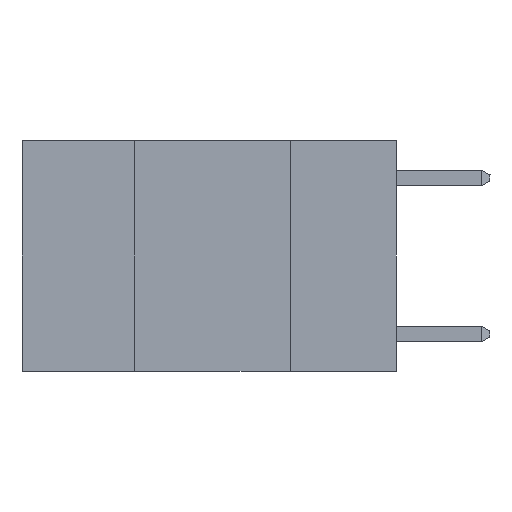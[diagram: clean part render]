
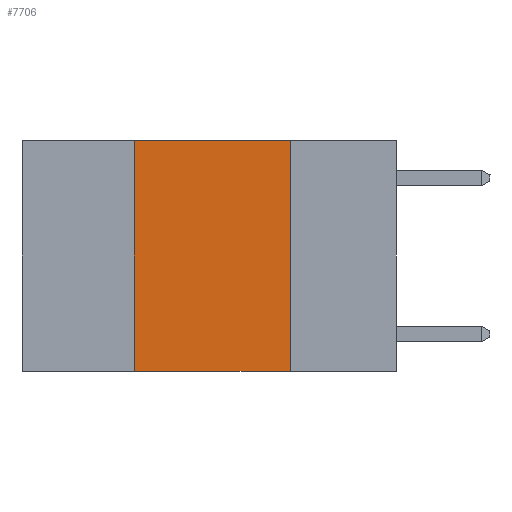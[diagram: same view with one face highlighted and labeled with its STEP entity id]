
A CAD part, left-side view. The second image highlights one B-rep face of the part: STEP entity #7706.
In plain terms, the highlighted planar face has unit normal (-1, 0, 0).
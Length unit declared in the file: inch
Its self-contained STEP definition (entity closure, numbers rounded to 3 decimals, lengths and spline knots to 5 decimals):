
#62 = ORIENTED_EDGE ( 'NONE', *, *, #2070, .F. ) ;
#86 = CARTESIAN_POINT ( 'NONE',  ( 0., 0.6, -0.37 ) ) ;
#140 = PLANE ( 'NONE',  #3904 ) ;
#459 = DIRECTION ( 'NONE',  ( 0., -1., 0. ) ) ;
#2070 = EDGE_CURVE ( 'NONE', #9289, #2929, #2936, .T. ) ;
#2397 = FACE_OUTER_BOUND ( 'NONE', #9527, .T. ) ;
#2909 = VECTOR ( 'NONE', #459, 39.37008 ) ;
#2929 = VERTEX_POINT ( 'NONE', #5144 ) ;
#2933 = CARTESIAN_POINT ( 'NONE',  ( 0., 0.6, 0. ) ) ;
#2936 = LINE ( 'NONE', #5142, #5556 ) ;
#3004 = EDGE_CURVE ( 'NONE', #8438, #9289, #6847, .T. ) ;
#3589 = EDGE_CURVE ( 'NONE', #9292, #2929, #6780, .T. ) ;
#3771 = DIRECTION ( 'NONE',  ( 0., 0., -1. ) ) ;
#3900 = DIRECTION ( 'NONE',  ( 0., -1., 0. ) ) ;
#3904 = AXIS2_PLACEMENT_3D ( 'NONE', #2933, #5977, #8201 ) ;
#3919 = ORIENTED_EDGE ( 'NONE', *, *, #3589, .T. ) ;
#4177 = ORIENTED_EDGE ( 'NONE', *, *, #8016, .F. ) ;
#4740 = CARTESIAN_POINT ( 'NONE',  ( 0., 0.6, 0. ) ) ;
#4844 = VECTOR ( 'NONE', #8734, 39.37008 ) ;
#5080 = CARTESIAN_POINT ( 'NONE',  ( 0., 0.17, 0. ) ) ;
#5142 = CARTESIAN_POINT ( 'NONE',  ( 0., 0.17, 0. ) ) ;
#5144 = CARTESIAN_POINT ( 'NONE',  ( 0., 0.17, -0.37 ) ) ;
#5285 = VECTOR ( 'NONE', #3900, 39.37008 ) ;
#5556 = VECTOR ( 'NONE', #3771, 39.37008 ) ;
#5977 = DIRECTION ( 'NONE',  ( 1., 0., 0. ) ) ;
#6107 = CARTESIAN_POINT ( 'NONE',  ( 0., 0.42, 0. ) ) ;
#6584 = CARTESIAN_POINT ( 'NONE',  ( 0., 0.42, 0. ) ) ;
#6780 = LINE ( 'NONE', #86, #2909 ) ;
#6847 = LINE ( 'NONE', #4740, #5285 ) ;
#6950 = ORIENTED_EDGE ( 'NONE', *, *, #3004, .F. ) ;
#7706 = ADVANCED_FACE ( 'NONE', ( #2397 ), #140, .F. ) ;
#8016 = EDGE_CURVE ( 'NONE', #9292, #8438, #9513, .T. ) ;
#8048 = CARTESIAN_POINT ( 'NONE',  ( 0., 0.42, -0.37 ) ) ;
#8201 = DIRECTION ( 'NONE',  ( 0., 0., -1. ) ) ;
#8438 = VERTEX_POINT ( 'NONE', #6107 ) ;
#8734 = DIRECTION ( 'NONE',  ( 0., 0., 1. ) ) ;
#9289 = VERTEX_POINT ( 'NONE', #5080 ) ;
#9292 = VERTEX_POINT ( 'NONE', #8048 ) ;
#9513 = LINE ( 'NONE', #6584, #4844 ) ;
#9527 = EDGE_LOOP ( 'NONE', ( #62, #6950, #4177, #3919 ) ) ;
